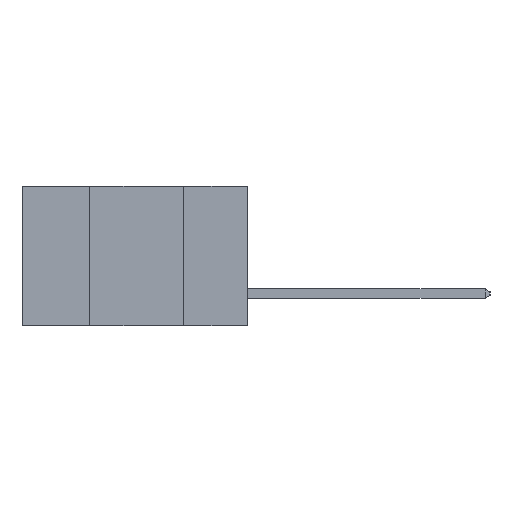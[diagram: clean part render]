
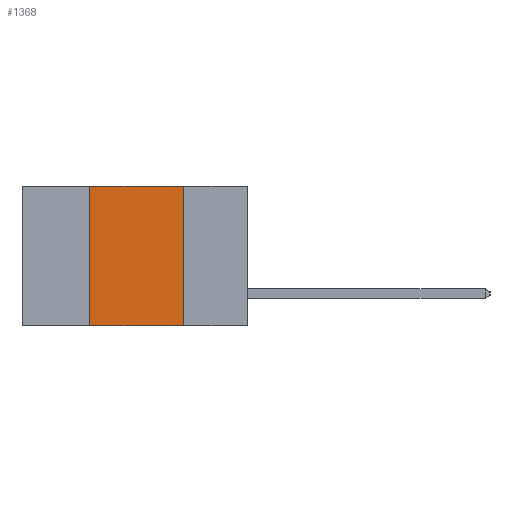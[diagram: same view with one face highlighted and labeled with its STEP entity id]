
A CAD part, left-side view. The second image highlights one B-rep face of the part: STEP entity #1368.
In plain terms, the highlighted planar face has unit normal (-1, 0, 0).
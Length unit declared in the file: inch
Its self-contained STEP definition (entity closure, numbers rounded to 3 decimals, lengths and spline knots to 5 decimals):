
#270 = VECTOR ( 'NONE', #17464, 39.37008 ) ;
#739 = EDGE_LOOP ( 'NONE', ( #5892, #15289, #15127, #802 ) ) ;
#753 = LINE ( 'NONE', #1000, #270 ) ;
#802 = ORIENTED_EDGE ( 'NONE', *, *, #11268, .T. ) ;
#942 = DIRECTION ( 'NONE',  ( 0., -1., 0. ) ) ;
#1000 = CARTESIAN_POINT ( 'NONE',  ( 0., 0.6, -0.37 ) ) ;
#1368 = ADVANCED_FACE ( 'NONE', ( #2992 ), #13746, .F. ) ;
#1590 = VECTOR ( 'NONE', #942, 39.37008 ) ;
#1627 = LINE ( 'NONE', #1884, #15440 ) ;
#1884 = CARTESIAN_POINT ( 'NONE',  ( 0., 0.17, -0.37 ) ) ;
#2351 = VERTEX_POINT ( 'NONE', #5096 ) ;
#2992 = FACE_OUTER_BOUND ( 'NONE', #739, .T. ) ;
#3089 = VERTEX_POINT ( 'NONE', #4323 ) ;
#4323 = CARTESIAN_POINT ( 'NONE',  ( 0., 0.17, -0.37 ) ) ;
#5096 = CARTESIAN_POINT ( 'NONE',  ( 0., 0.42, 0. ) ) ;
#5892 = ORIENTED_EDGE ( 'NONE', *, *, #7504, .F. ) ;
#6180 = VERTEX_POINT ( 'NONE', #12788 ) ;
#7504 = EDGE_CURVE ( 'NONE', #17380, #3089, #1627, .T. ) ;
#7528 = AXIS2_PLACEMENT_3D ( 'NONE', #13991, #13725, #13710 ) ;
#8282 = VECTOR ( 'NONE', #13154, 39.37008 ) ;
#8381 = EDGE_CURVE ( 'NONE', #2351, #17380, #15007, .T. ) ;
#8964 = DIRECTION ( 'NONE',  ( 0., 0., -1. ) ) ;
#11049 = EDGE_CURVE ( 'NONE', #6180, #2351, #15735, .T. ) ;
#11268 = EDGE_CURVE ( 'NONE', #6180, #3089, #753, .T. ) ;
#11429 = CARTESIAN_POINT ( 'NONE',  ( 0., 0.17, 0. ) ) ;
#11820 = CARTESIAN_POINT ( 'NONE',  ( 0., 0.42, -0.37 ) ) ;
#12788 = CARTESIAN_POINT ( 'NONE',  ( 0., 0.42, -0.37 ) ) ;
#13154 = DIRECTION ( 'NONE',  ( 0., 0., 1. ) ) ;
#13710 = DIRECTION ( 'NONE',  ( 0., 0., -1. ) ) ;
#13725 = DIRECTION ( 'NONE',  ( 1., 0., 0. ) ) ;
#13746 = PLANE ( 'NONE',  #7528 ) ;
#13991 = CARTESIAN_POINT ( 'NONE',  ( 0., 0.6, 0. ) ) ;
#15007 = LINE ( 'NONE', #17404, #1590 ) ;
#15127 = ORIENTED_EDGE ( 'NONE', *, *, #11049, .F. ) ;
#15289 = ORIENTED_EDGE ( 'NONE', *, *, #8381, .F. ) ;
#15440 = VECTOR ( 'NONE', #8964, 39.37008 ) ;
#15735 = LINE ( 'NONE', #11820, #8282 ) ;
#17380 = VERTEX_POINT ( 'NONE', #11429 ) ;
#17404 = CARTESIAN_POINT ( 'NONE',  ( 0., 0.6, 0. ) ) ;
#17464 = DIRECTION ( 'NONE',  ( 0., -1., 0. ) ) ;
